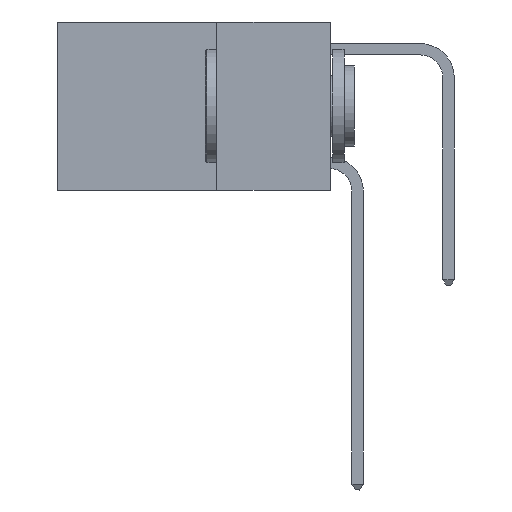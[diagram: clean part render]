
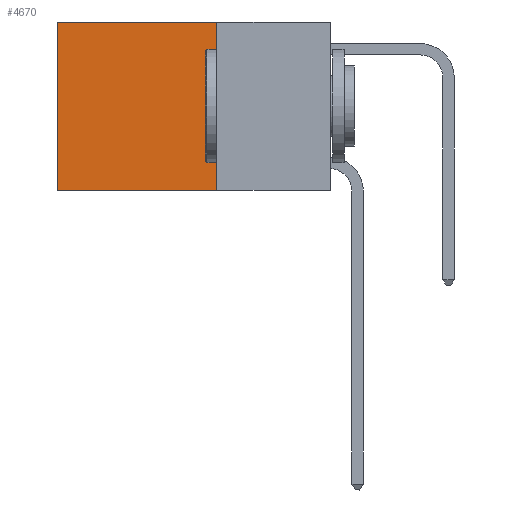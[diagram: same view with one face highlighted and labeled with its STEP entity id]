
A CAD part, left-side view. The second image highlights one B-rep face of the part: STEP entity #4670.
In plain terms, the highlighted planar face has unit normal (-1, 0, 0).
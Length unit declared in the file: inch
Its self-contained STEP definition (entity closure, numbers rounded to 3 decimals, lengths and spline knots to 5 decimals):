
#443 = LINE ( 'NONE', #7760, #13478 ) ;
#776 = EDGE_LOOP ( 'NONE', ( #7785, #16464, #15447, #8332 ) ) ;
#794 = DIRECTION ( 'NONE',  ( 1., 0., 0. ) ) ;
#1000 = DIRECTION ( 'NONE',  ( 0., 0., -1. ) ) ;
#1484 = VERTEX_POINT ( 'NONE', #15752 ) ;
#2527 = VERTEX_POINT ( 'NONE', #20166 ) ;
#3816 = AXIS2_PLACEMENT_3D ( 'NONE', #15907, #794, #9073 ) ;
#4670 = ADVANCED_FACE ( 'NONE', ( #5709 ), #15762, .F. ) ;
#4729 = EDGE_CURVE ( 'NONE', #15738, #2527, #443, .T. ) ;
#5103 = CARTESIAN_POINT ( 'NONE',  ( 0.2625, 0.6, 0. ) ) ;
#5233 = EDGE_CURVE ( 'NONE', #21572, #1484, #13204, .T. ) ;
#5709 = FACE_OUTER_BOUND ( 'NONE', #776, .T. ) ;
#6955 = CARTESIAN_POINT ( 'NONE',  ( 0.2625, 0.25, -0.37 ) ) ;
#7705 = VECTOR ( 'NONE', #17505, 39.37008 ) ;
#7760 = CARTESIAN_POINT ( 'NONE',  ( 0.2625, 0.6, 0. ) ) ;
#7785 = ORIENTED_EDGE ( 'NONE', *, *, #4729, .T. ) ;
#8332 = ORIENTED_EDGE ( 'NONE', *, *, #11217, .T. ) ;
#8694 = CARTESIAN_POINT ( 'NONE',  ( 0.2625, 0.25, 0. ) ) ;
#8736 = LINE ( 'NONE', #16628, #18094 ) ;
#9073 = DIRECTION ( 'NONE',  ( 0., 0., -1. ) ) ;
#11217 = EDGE_CURVE ( 'NONE', #21572, #15738, #8736, .T. ) ;
#11407 = EDGE_CURVE ( 'NONE', #1484, #2527, #18614, .T. ) ;
#12695 = VECTOR ( 'NONE', #1000, 39.37008 ) ;
#13204 = LINE ( 'NONE', #8694, #12695 ) ;
#13478 = VECTOR ( 'NONE', #17865, 39.37008 ) ;
#15122 = CARTESIAN_POINT ( 'NONE',  ( 0.2625, 0.25, 0. ) ) ;
#15447 = ORIENTED_EDGE ( 'NONE', *, *, #5233, .F. ) ;
#15738 = VERTEX_POINT ( 'NONE', #5103 ) ;
#15752 = CARTESIAN_POINT ( 'NONE',  ( 0.2625, 0.25, -0.37 ) ) ;
#15762 = PLANE ( 'NONE',  #3816 ) ;
#15907 = CARTESIAN_POINT ( 'NONE',  ( 0.2625, 0.25, 0. ) ) ;
#16464 = ORIENTED_EDGE ( 'NONE', *, *, #11407, .F. ) ;
#16628 = CARTESIAN_POINT ( 'NONE',  ( 0.2625, 0.25, 0. ) ) ;
#17505 = DIRECTION ( 'NONE',  ( 0., 1., 0. ) ) ;
#17865 = DIRECTION ( 'NONE',  ( 0., 0., -1. ) ) ;
#18094 = VECTOR ( 'NONE', #18526, 39.37008 ) ;
#18526 = DIRECTION ( 'NONE',  ( 0., 1., 0. ) ) ;
#18614 = LINE ( 'NONE', #6955, #7705 ) ;
#20166 = CARTESIAN_POINT ( 'NONE',  ( 0.2625, 0.6, -0.37 ) ) ;
#21572 = VERTEX_POINT ( 'NONE', #15122 ) ;
